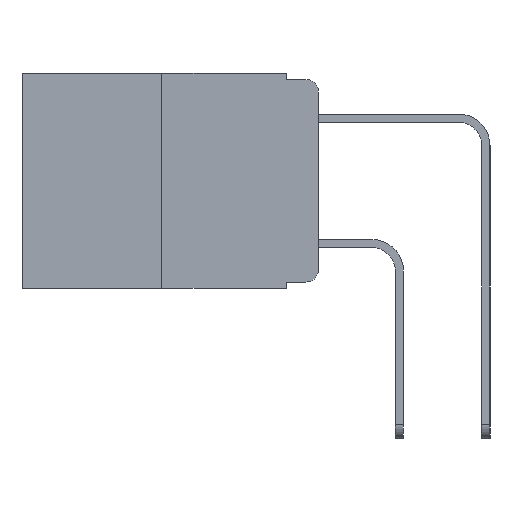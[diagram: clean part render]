
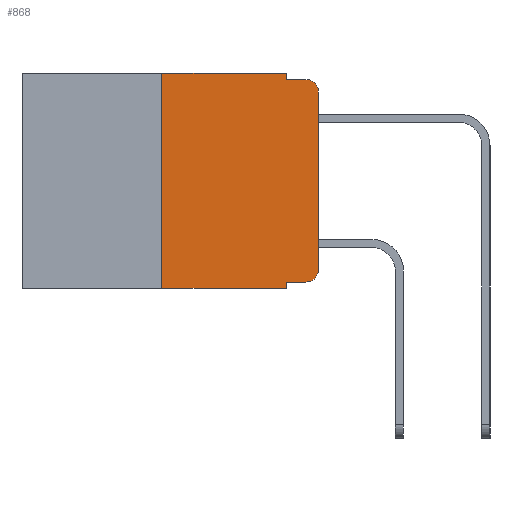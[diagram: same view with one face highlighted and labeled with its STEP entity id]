
A CAD part, left-side view. The second image highlights one B-rep face of the part: STEP entity #868.
In plain terms, the highlighted planar face has unit normal (-1, 0, 0).
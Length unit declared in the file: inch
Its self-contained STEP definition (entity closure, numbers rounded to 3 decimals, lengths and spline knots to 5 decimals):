
#33 = CARTESIAN_POINT ( 'NONE',  ( 0., 0.473, -0.343 ) ) ;
#165 = VERTEX_POINT ( 'NONE', #2082 ) ;
#331 = ORIENTED_EDGE ( 'NONE', *, *, #6346, .T. ) ;
#519 = LINE ( 'NONE', #17318, #14600 ) ;
#868 = ADVANCED_FACE ( 'NONE', ( #5905 ), #17023, .F. ) ;
#871 = AXIS2_PLACEMENT_3D ( 'NONE', #17089, #16978, #16957 ) ;
#887 = ORIENTED_EDGE ( 'NONE', *, *, #8149, .T. ) ;
#1005 = CARTESIAN_POINT ( 'NONE',  ( 0., 0.051, 0. ) ) ;
#1208 = AXIS2_PLACEMENT_3D ( 'NONE', #1701, #11352, #3162 ) ;
#1377 = CARTESIAN_POINT ( 'NONE',  ( 0., 0.25, -0.343 ) ) ;
#1701 = CARTESIAN_POINT ( 'NONE',  ( 0., 0.02, -0.313 ) ) ;
#1772 = LINE ( 'NONE', #6053, #8323 ) ;
#1856 = ORIENTED_EDGE ( 'NONE', *, *, #4508, .F. ) ;
#1942 = LINE ( 'NONE', #5547, #5309 ) ;
#2038 = CIRCLE ( 'NONE', #1208, 0.02 ) ;
#2082 = CARTESIAN_POINT ( 'NONE',  ( 0., 0.051, -0.333 ) ) ;
#2090 = VERTEX_POINT ( 'NONE', #9345 ) ;
#2478 = VECTOR ( 'NONE', #14188, 39.37008 ) ;
#2546 = EDGE_CURVE ( 'NONE', #11892, #17454, #1942, .T. ) ;
#2636 = VECTOR ( 'NONE', #7712, 39.37008 ) ;
#2680 = CARTESIAN_POINT ( 'NONE',  ( 0., 0.02, -0.03 ) ) ;
#2906 = LINE ( 'NONE', #1005, #5350 ) ;
#2944 = LINE ( 'NONE', #16749, #2478 ) ;
#3162 = DIRECTION ( 'NONE',  ( 0., 0., -1. ) ) ;
#3426 = VECTOR ( 'NONE', #11119, 39.37008 ) ;
#4052 = VECTOR ( 'NONE', #14814, 39.37008 ) ;
#4136 = DIRECTION ( 'NONE',  ( 0., 0., -1. ) ) ;
#4430 = ORIENTED_EDGE ( 'NONE', *, *, #17219, .F. ) ;
#4497 = LINE ( 'NONE', #5543, #4052 ) ;
#4508 = EDGE_CURVE ( 'NONE', #17454, #7773, #519, .T. ) ;
#4858 = ORIENTED_EDGE ( 'NONE', *, *, #2546, .F. ) ;
#5309 = VECTOR ( 'NONE', #8099, 39.37008 ) ;
#5350 = VECTOR ( 'NONE', #8053, 39.37008 ) ;
#5500 = CARTESIAN_POINT ( 'NONE',  ( 0., 0.051, -0.01 ) ) ;
#5543 = CARTESIAN_POINT ( 'NONE',  ( 0., 0., 0. ) ) ;
#5547 = CARTESIAN_POINT ( 'NONE',  ( 0., 0.051, 0. ) ) ;
#5905 = FACE_OUTER_BOUND ( 'NONE', #7299, .T. ) ;
#6053 = CARTESIAN_POINT ( 'NONE',  ( 0., 0.473, 0. ) ) ;
#6252 = CIRCLE ( 'NONE', #7287, 0.02 ) ;
#6346 = EDGE_CURVE ( 'NONE', #11704, #7773, #6252, .T. ) ;
#6604 = CARTESIAN_POINT ( 'NONE',  ( 0., 0.25, 0. ) ) ;
#7022 = VERTEX_POINT ( 'NONE', #1377 ) ;
#7287 = AXIS2_PLACEMENT_3D ( 'NONE', #2680, #12233, #4136 ) ;
#7299 = EDGE_LOOP ( 'NONE', ( #887, #331, #1856, #4858, #8915, #4430, #8959, #7606, #11658, #10078 ) ) ;
#7606 = ORIENTED_EDGE ( 'NONE', *, *, #15518, .F. ) ;
#7619 = CARTESIAN_POINT ( 'NONE',  ( 0., 0.051, -0.343 ) ) ;
#7712 = DIRECTION ( 'NONE',  ( 0., 0., 1. ) ) ;
#7773 = VERTEX_POINT ( 'NONE', #12711 ) ;
#8053 = DIRECTION ( 'NONE',  ( 0., 0., -1. ) ) ;
#8099 = DIRECTION ( 'NONE',  ( 0., 0., -1. ) ) ;
#8149 = EDGE_CURVE ( 'NONE', #9532, #11704, #4497, .T. ) ;
#8320 = CARTESIAN_POINT ( 'NONE',  ( 0., 0., -0.313 ) ) ;
#8323 = VECTOR ( 'NONE', #15249, 39.37008 ) ;
#8619 = VERTEX_POINT ( 'NONE', #6604 ) ;
#8915 = ORIENTED_EDGE ( 'NONE', *, *, #15325, .F. ) ;
#8959 = ORIENTED_EDGE ( 'NONE', *, *, #11961, .T. ) ;
#9198 = CARTESIAN_POINT ( 'NONE',  ( 0., 0., -0.03 ) ) ;
#9345 = CARTESIAN_POINT ( 'NONE',  ( 0., 0.02, -0.333 ) ) ;
#9532 = VERTEX_POINT ( 'NONE', #8320 ) ;
#9549 = DIRECTION ( 'NONE',  ( 0., -1., 0. ) ) ;
#10078 = ORIENTED_EDGE ( 'NONE', *, *, #12073, .T. ) ;
#11119 = DIRECTION ( 'NONE',  ( 0., -1., 0. ) ) ;
#11352 = DIRECTION ( 'NONE',  ( -1., 0., 0. ) ) ;
#11658 = ORIENTED_EDGE ( 'NONE', *, *, #14658, .T. ) ;
#11704 = VERTEX_POINT ( 'NONE', #9198 ) ;
#11892 = VERTEX_POINT ( 'NONE', #14798 ) ;
#11961 = EDGE_CURVE ( 'NONE', #7022, #16556, #14566, .T. ) ;
#12073 = EDGE_CURVE ( 'NONE', #2090, #9532, #2038, .T. ) ;
#12233 = DIRECTION ( 'NONE',  ( -1., 0., 0. ) ) ;
#12711 = CARTESIAN_POINT ( 'NONE',  ( 0., 0.02, -0.01 ) ) ;
#14188 = DIRECTION ( 'NONE',  ( 0., -1., 0. ) ) ;
#14566 = LINE ( 'NONE', #33, #3426 ) ;
#14600 = VECTOR ( 'NONE', #9549, 39.37008 ) ;
#14658 = EDGE_CURVE ( 'NONE', #165, #2090, #2944, .T. ) ;
#14798 = CARTESIAN_POINT ( 'NONE',  ( 0., 0.051, 0. ) ) ;
#14814 = DIRECTION ( 'NONE',  ( 0., 0., 1. ) ) ;
#15249 = DIRECTION ( 'NONE',  ( 0., -1., 0. ) ) ;
#15325 = EDGE_CURVE ( 'NONE', #8619, #11892, #1772, .T. ) ;
#15518 = EDGE_CURVE ( 'NONE', #165, #16556, #2906, .T. ) ;
#15583 = CARTESIAN_POINT ( 'NONE',  ( 0., 0.25, 0. ) ) ;
#16058 = LINE ( 'NONE', #15583, #2636 ) ;
#16556 = VERTEX_POINT ( 'NONE', #7619 ) ;
#16749 = CARTESIAN_POINT ( 'NONE',  ( 0., 0.051, -0.333 ) ) ;
#16957 = DIRECTION ( 'NONE',  ( 0., 0., -1. ) ) ;
#16978 = DIRECTION ( 'NONE',  ( 1., 0., 0. ) ) ;
#17023 = PLANE ( 'NONE',  #871 ) ;
#17089 = CARTESIAN_POINT ( 'NONE',  ( 0., 0.473, 0. ) ) ;
#17219 = EDGE_CURVE ( 'NONE', #7022, #8619, #16058, .T. ) ;
#17318 = CARTESIAN_POINT ( 'NONE',  ( 0., 0.051, -0.01 ) ) ;
#17454 = VERTEX_POINT ( 'NONE', #5500 ) ;
